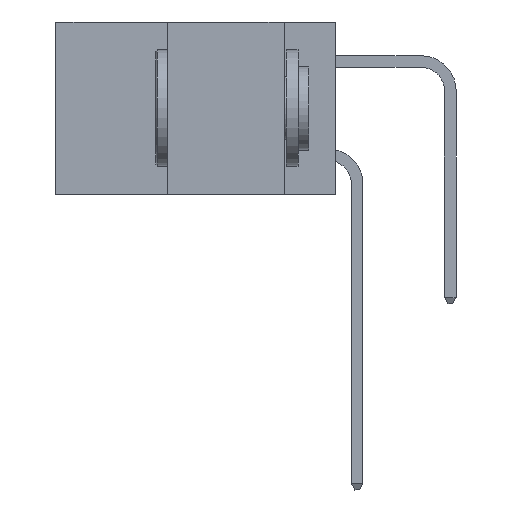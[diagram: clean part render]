
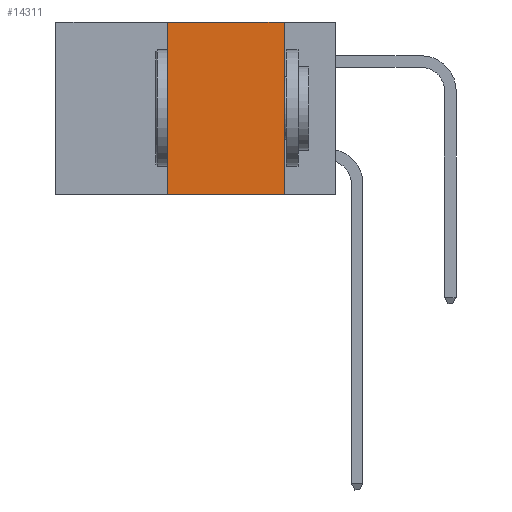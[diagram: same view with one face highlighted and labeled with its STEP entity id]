
A CAD part, left-side view. The second image highlights one B-rep face of the part: STEP entity #14311.
In plain terms, the highlighted planar face has unit normal (-1, 0, 0).
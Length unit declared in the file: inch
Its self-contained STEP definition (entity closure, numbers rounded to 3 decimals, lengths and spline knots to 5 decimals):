
#1507 = LINE ( 'NONE', #23544, #23812 ) ;
#2831 = CARTESIAN_POINT ( 'NONE',  ( 0., 0.36, 0. ) ) ;
#3016 = DIRECTION ( 'NONE',  ( 0., -1., 0. ) ) ;
#3990 = EDGE_CURVE ( 'NONE', #13910, #24827, #5730, .T. ) ;
#4211 = VECTOR ( 'NONE', #25282, 39.37008 ) ;
#5730 = LINE ( 'NONE', #14610, #16858 ) ;
#5922 = FACE_OUTER_BOUND ( 'NONE', #23854, .T. ) ;
#6143 = CARTESIAN_POINT ( 'NONE',  ( 0., 0.36, -0.37 ) ) ;
#6585 = DIRECTION ( 'NONE',  ( 0., 0., -1. ) ) ;
#8131 = ORIENTED_EDGE ( 'NONE', *, *, #14546, .F. ) ;
#9051 = CARTESIAN_POINT ( 'NONE',  ( 0., 0.6, 0. ) ) ;
#10550 = AXIS2_PLACEMENT_3D ( 'NONE', #9051, #11538, #28132 ) ;
#10691 = VERTEX_POINT ( 'NONE', #6143 ) ;
#11212 = EDGE_CURVE ( 'NONE', #10691, #13910, #11253, .T. ) ;
#11253 = LINE ( 'NONE', #13317, #4211 ) ;
#11485 = VERTEX_POINT ( 'NONE', #14068 ) ;
#11538 = DIRECTION ( 'NONE',  ( 1., 0., 0. ) ) ;
#13317 = CARTESIAN_POINT ( 'NONE',  ( 0., 0.36, 0. ) ) ;
#13663 = EDGE_CURVE ( 'NONE', #10691, #11485, #1507, .T. ) ;
#13910 = VERTEX_POINT ( 'NONE', #2831 ) ;
#14029 = PLANE ( 'NONE',  #10550 ) ;
#14068 = CARTESIAN_POINT ( 'NONE',  ( 0., 0.11, -0.37 ) ) ;
#14311 = ADVANCED_FACE ( 'NONE', ( #5922 ), #14029, .F. ) ;
#14546 = EDGE_CURVE ( 'NONE', #24827, #11485, #18943, .T. ) ;
#14610 = CARTESIAN_POINT ( 'NONE',  ( 0., 0.6, 0. ) ) ;
#16745 = ORIENTED_EDGE ( 'NONE', *, *, #11212, .F. ) ;
#16858 = VECTOR ( 'NONE', #3016, 39.37008 ) ;
#16876 = CARTESIAN_POINT ( 'NONE',  ( 0., 0.11, 0. ) ) ;
#18943 = LINE ( 'NONE', #23428, #30119 ) ;
#19454 = ORIENTED_EDGE ( 'NONE', *, *, #13663, .T. ) ;
#23428 = CARTESIAN_POINT ( 'NONE',  ( 0., 0.11, 0. ) ) ;
#23544 = CARTESIAN_POINT ( 'NONE',  ( 0., 0.6, -0.37 ) ) ;
#23812 = VECTOR ( 'NONE', #26242, 39.37008 ) ;
#23854 = EDGE_LOOP ( 'NONE', ( #8131, #24021, #16745, #19454 ) ) ;
#24021 = ORIENTED_EDGE ( 'NONE', *, *, #3990, .F. ) ;
#24827 = VERTEX_POINT ( 'NONE', #16876 ) ;
#25282 = DIRECTION ( 'NONE',  ( 0., 0., 1. ) ) ;
#26242 = DIRECTION ( 'NONE',  ( 0., -1., 0. ) ) ;
#28132 = DIRECTION ( 'NONE',  ( 0., 0., -1. ) ) ;
#30119 = VECTOR ( 'NONE', #6585, 39.37008 ) ;
